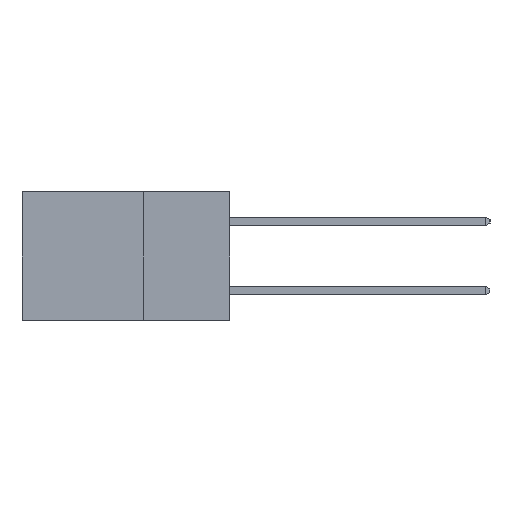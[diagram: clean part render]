
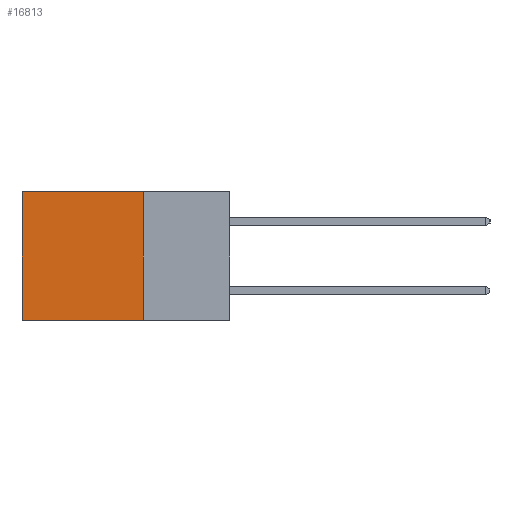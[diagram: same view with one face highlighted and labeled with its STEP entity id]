
A CAD part, left-side view. The second image highlights one B-rep face of the part: STEP entity #16813.
In plain terms, the highlighted planar face has unit normal (-1, 0, 0).
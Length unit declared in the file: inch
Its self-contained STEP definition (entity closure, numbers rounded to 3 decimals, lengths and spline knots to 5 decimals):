
#370 = VERTEX_POINT ( 'NONE', #23822 ) ;
#810 = ORIENTED_EDGE ( 'NONE', *, *, #18797, .T. ) ;
#2649 = CARTESIAN_POINT ( 'NONE',  ( 0.2615, 0.25, 0. ) ) ;
#4025 = CARTESIAN_POINT ( 'NONE',  ( 0.2615, 0.25, -0.37 ) ) ;
#4983 = ORIENTED_EDGE ( 'NONE', *, *, #16165, .T. ) ;
#5923 = DIRECTION ( 'NONE',  ( 0., 0., -1. ) ) ;
#6737 = VECTOR ( 'NONE', #7938, 39.37008 ) ;
#7331 = LINE ( 'NONE', #17114, #6737 ) ;
#7938 = DIRECTION ( 'NONE',  ( 0., 1., 0. ) ) ;
#8388 = LINE ( 'NONE', #9850, #16990 ) ;
#9850 = CARTESIAN_POINT ( 'NONE',  ( 0.2615, 0.25, -0.37 ) ) ;
#9930 = EDGE_CURVE ( 'NONE', #14109, #17914, #7331, .T. ) ;
#10241 = LINE ( 'NONE', #22735, #19436 ) ;
#12164 = ORIENTED_EDGE ( 'NONE', *, *, #9930, .F. ) ;
#13149 = DIRECTION ( 'NONE',  ( 0., 1., 0. ) ) ;
#13377 = PLANE ( 'NONE',  #22059 ) ;
#13590 = DIRECTION ( 'NONE',  ( 0., 0., -1. ) ) ;
#14109 = VERTEX_POINT ( 'NONE', #20476 ) ;
#14454 = ORIENTED_EDGE ( 'NONE', *, *, #18287, .F. ) ;
#14455 = CARTESIAN_POINT ( 'NONE',  ( 0.2615, 0.6, -0.37 ) ) ;
#14663 = EDGE_LOOP ( 'NONE', ( #810, #12164, #14454, #4983 ) ) ;
#16165 = EDGE_CURVE ( 'NONE', #18939, #370, #19395, .T. ) ;
#16813 = ADVANCED_FACE ( 'NONE', ( #23946 ), #13377, .F. ) ;
#16990 = VECTOR ( 'NONE', #19080, 39.37008 ) ;
#17021 = DIRECTION ( 'NONE',  ( 1., 0., 0. ) ) ;
#17114 = CARTESIAN_POINT ( 'NONE',  ( 0.2615, 0.25, -0.37 ) ) ;
#17914 = VERTEX_POINT ( 'NONE', #14455 ) ;
#18287 = EDGE_CURVE ( 'NONE', #18939, #14109, #8388, .T. ) ;
#18797 = EDGE_CURVE ( 'NONE', #370, #17914, #10241, .T. ) ;
#18939 = VERTEX_POINT ( 'NONE', #2649 ) ;
#19080 = DIRECTION ( 'NONE',  ( 0., 0., -1. ) ) ;
#19395 = LINE ( 'NONE', #23562, #23689 ) ;
#19436 = VECTOR ( 'NONE', #13590, 39.37008 ) ;
#20476 = CARTESIAN_POINT ( 'NONE',  ( 0.2615, 0.25, -0.37 ) ) ;
#22059 = AXIS2_PLACEMENT_3D ( 'NONE', #4025, #17021, #5923 ) ;
#22735 = CARTESIAN_POINT ( 'NONE',  ( 0.2615, 0.6, -0.37 ) ) ;
#23562 = CARTESIAN_POINT ( 'NONE',  ( 0.2615, 0.25, 0. ) ) ;
#23689 = VECTOR ( 'NONE', #13149, 39.37008 ) ;
#23822 = CARTESIAN_POINT ( 'NONE',  ( 0.2615, 0.6, 0. ) ) ;
#23946 = FACE_OUTER_BOUND ( 'NONE', #14663, .T. ) ;
